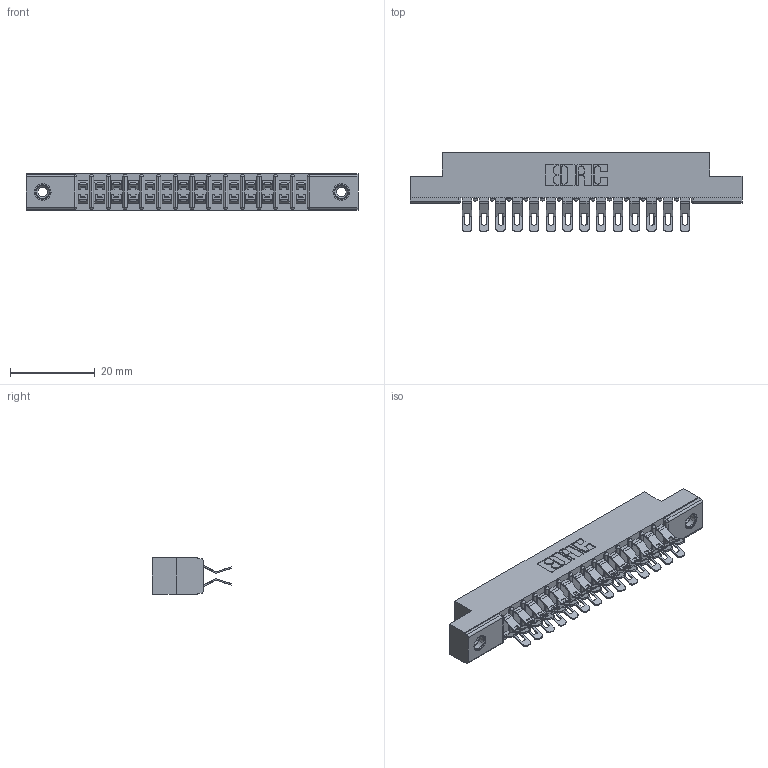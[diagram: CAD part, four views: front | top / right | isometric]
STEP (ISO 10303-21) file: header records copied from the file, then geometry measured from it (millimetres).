
FILE_DESCRIPTION (( 'STEP AP203' ), '1' );
FILE_NAME ('357-028-555-208.STEP', '2019-09-17T23:49:48', ( '' ), ( '' ), 'SwSTEP 2.0', 'SolidWorks 2016', '' );
FILE_SCHEMA (( 'CONFIG_CONTROL_DESIGN' ));
Length unit declared in the file: inch
Products named in the file (4): 345-250-001_345-250-003-102; 357-028-555-208; 307-290-001_555; 307 Part_.156 Dia Mounting Holes
Assembly tree (31 placements, depth 2):
  357-028-555-208
    307 Part_.156 Dia Mounting Holes
    307-290-001_555  x28
    345-250-001_345-250-003-102  x2
Bounding box: 78.49 x 18.75 x 8.71 mm (x, y, z)
Volume: 5211.6 mm3; surface area: 9270.2 mm2
Topology: 31 solids, 31 shells, 1901 faces, 5527 edges, 3598 vertices
Faces by surface type: plane 1054, cylinder 801, sphere 30, cone 12, torus 4
Entity records: 17624 total; most frequent: CARTESIAN_POINT 2881, DIRECTION 2850, ORIENTED_EDGE 2848, EDGE_CURVE 1424, LINE 1068, VECTOR 1068, VERTEX_POINT 922, AXIS2_PLACEMENT_3D 891
